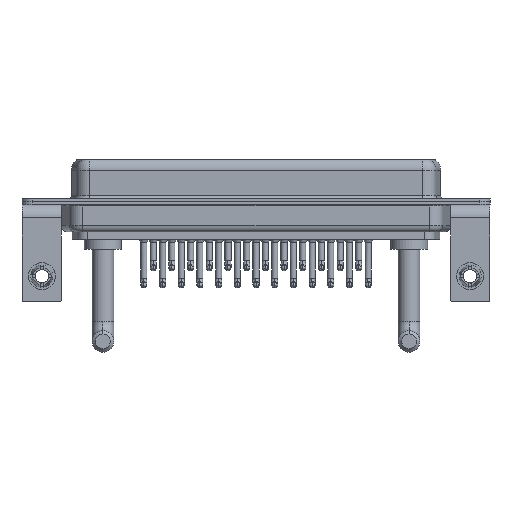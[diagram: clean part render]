
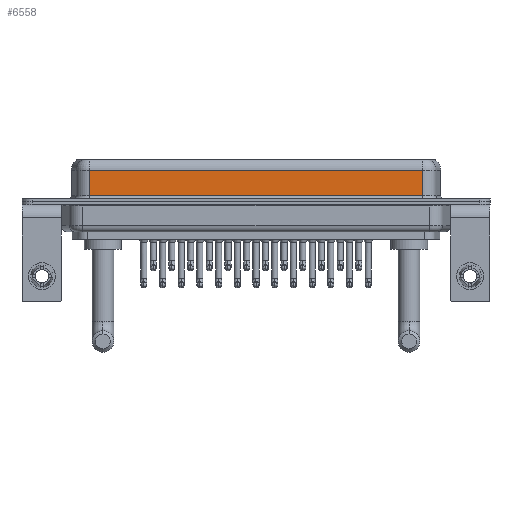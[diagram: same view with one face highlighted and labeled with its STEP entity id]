
A CAD part, front view. The second image highlights one B-rep face of the part: STEP entity #6558.
In plain terms, the highlighted planar face has unit normal (0, -1, 0).
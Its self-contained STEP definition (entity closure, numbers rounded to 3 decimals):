
#738 = VECTOR ( 'NONE', #20576, 1000. ) ;
#962 = DIRECTION ( 'NONE',  ( -1., 0., 0. ) ) ;
#1020 = FACE_OUTER_BOUND ( 'NONE', #24380, .T. ) ;
#2136 = VERTEX_POINT ( 'NONE', #23092 ) ;
#4649 = VERTEX_POINT ( 'NONE', #24931 ) ;
#5132 = CARTESIAN_POINT ( 'NONE',  ( 56.462, -3.95, 6.4 ) ) ;
#5161 = CARTESIAN_POINT ( 'NONE',  ( 56.462, -3.95, 6.4 ) ) ;
#5263 = VERTEX_POINT ( 'NONE', #22596 ) ;
#5402 = VERTEX_POINT ( 'NONE', #23406 ) ;
#5505 = CARTESIAN_POINT ( 'NONE',  ( 56.462, -3.95, 4.65 ) ) ;
#6558 = ADVANCED_FACE ( 'NONE', ( #1020 ), #23476, .F. ) ;
#7936 = LINE ( 'NONE', #24710, #738 ) ;
#9146 = DIRECTION ( 'NONE',  ( 0., 0., -1. ) ) ;
#9312 = EDGE_CURVE ( 'NONE', #2136, #5402, #7936, .T. ) ;
#9427 = DIRECTION ( 'NONE',  ( 0., 0., 1. ) ) ;
#10099 = EDGE_CURVE ( 'NONE', #5263, #5402, #17797, .T. ) ;
#11797 = LINE ( 'NONE', #13714, #14524 ) ;
#13568 = DIRECTION ( 'NONE',  ( 0., 1., 0. ) ) ;
#13714 = CARTESIAN_POINT ( 'NONE',  ( 7.038, -3.95, 6.4 ) ) ;
#14268 = ORIENTED_EDGE ( 'NONE', *, *, #22938, .T. ) ;
#14524 = VECTOR ( 'NONE', #16172, 1000. ) ;
#15812 = EDGE_CURVE ( 'NONE', #5263, #4649, #19811, .T. ) ;
#16172 = DIRECTION ( 'NONE',  ( 0., 0., -1. ) ) ;
#17377 = VECTOR ( 'NONE', #9146, 1000. ) ;
#17797 = LINE ( 'NONE', #5132, #17377 ) ;
#17888 = ORIENTED_EDGE ( 'NONE', *, *, #15812, .T. ) ;
#19385 = AXIS2_PLACEMENT_3D ( 'NONE', #5161, #13568, #9427 ) ;
#19811 = LINE ( 'NONE', #5505, #25574 ) ;
#20576 = DIRECTION ( 'NONE',  ( 1., 0., 0. ) ) ;
#22596 = CARTESIAN_POINT ( 'NONE',  ( 56.462, -3.95, 4.65 ) ) ;
#22922 = ORIENTED_EDGE ( 'NONE', *, *, #9312, .T. ) ;
#22938 = EDGE_CURVE ( 'NONE', #4649, #2136, #11797, .T. ) ;
#22965 = ORIENTED_EDGE ( 'NONE', *, *, #10099, .F. ) ;
#23092 = CARTESIAN_POINT ( 'NONE',  ( 7.038, -3.95, 0.9 ) ) ;
#23406 = CARTESIAN_POINT ( 'NONE',  ( 56.462, -3.95, 0.9 ) ) ;
#23476 = PLANE ( 'NONE',  #19385 ) ;
#24380 = EDGE_LOOP ( 'NONE', ( #22965, #17888, #14268, #22922 ) ) ;
#24710 = CARTESIAN_POINT ( 'NONE',  ( 56.462, -3.95, 0.9 ) ) ;
#24931 = CARTESIAN_POINT ( 'NONE',  ( 7.038, -3.95, 4.65 ) ) ;
#25574 = VECTOR ( 'NONE', #962, 1000. ) ;
